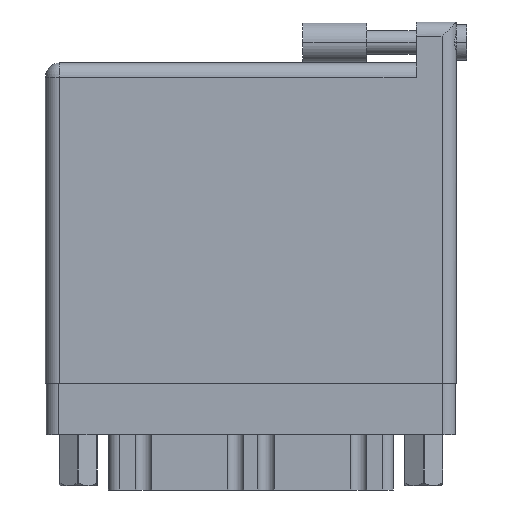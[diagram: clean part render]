
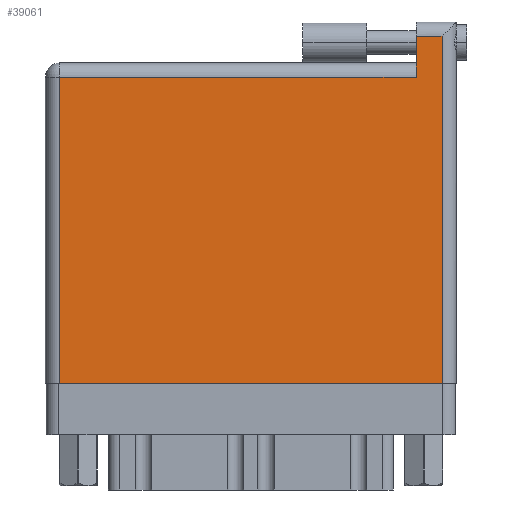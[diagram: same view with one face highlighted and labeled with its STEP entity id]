
A CAD part, front view. The second image highlights one B-rep face of the part: STEP entity #39061.
In plain terms, the highlighted face is planar.
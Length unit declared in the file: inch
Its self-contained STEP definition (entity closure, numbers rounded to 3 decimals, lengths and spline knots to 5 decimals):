
#5 = ORIENTED_EDGE ( 'NONE', *, *, #36815, .T. ) ;
#1291 = VERTEX_POINT ( 'NONE', #3061 ) ;
#2161 = VECTOR ( 'NONE', #46691, 39.37008 ) ;
#2641 = DIRECTION ( 'NONE',  ( -1., 0., 0. ) ) ;
#2986 = VECTOR ( 'NONE', #26670, 39.37008 ) ;
#3061 = CARTESIAN_POINT ( 'NONE',  ( 1.811, 1.496, 0. ) ) ;
#4085 = EDGE_CURVE ( 'NONE', #36814, #37633, #35829, .T. ) ;
#4167 = VERTEX_POINT ( 'NONE', #31505 ) ;
#5212 = EDGE_CURVE ( 'NONE', #37633, #35950, #10649, .T. ) ;
#6495 = ORIENTED_EDGE ( 'NONE', *, *, #18965, .T. ) ;
#6812 = CARTESIAN_POINT ( 'NONE',  ( 0., 0., 0. ) ) ;
#10148 = LINE ( 'NONE', #13484, #28667 ) ;
#10649 = LINE ( 'NONE', #6812, #2161 ) ;
#13034 = ORIENTED_EDGE ( 'NONE', *, *, #5212, .T. ) ;
#13484 = CARTESIAN_POINT ( 'NONE',  ( 1.938, 1.766, 0. ) ) ;
#13700 = LINE ( 'NONE', #32299, #39753 ) ;
#17679 = FACE_OUTER_BOUND ( 'NONE', #38819, .T. ) ;
#18419 = LINE ( 'NONE', #33679, #44116 ) ;
#18526 = EDGE_CURVE ( 'NONE', #35950, #4167, #10148, .T. ) ;
#18965 = EDGE_CURVE ( 'NONE', #1291, #36814, #13700, .T. ) ;
#19088 = CARTESIAN_POINT ( 'NONE',  ( 0.07, 0., 0. ) ) ;
#19485 = LINE ( 'NONE', #23302, #2986 ) ;
#21342 = DIRECTION ( 'NONE',  ( 0., 1., 0. ) ) ;
#23302 = CARTESIAN_POINT ( 'NONE',  ( 0., 1.696, 0. ) ) ;
#26670 = DIRECTION ( 'NONE',  ( -1., 0., 0. ) ) ;
#27756 = DIRECTION ( 'NONE',  ( -1., 0., 0. ) ) ;
#28126 = VERTEX_POINT ( 'NONE', #35622 ) ;
#28667 = VECTOR ( 'NONE', #21342, 39.37008 ) ;
#31330 = AXIS2_PLACEMENT_3D ( 'NONE', #43005, #46364, #2641 ) ;
#31355 = ORIENTED_EDGE ( 'NONE', *, *, #35654, .T. ) ;
#31505 = CARTESIAN_POINT ( 'NONE',  ( 1.938, 1.696, 0. ) ) ;
#32004 = DIRECTION ( 'NONE',  ( 0., -1., 0. ) ) ;
#32299 = CARTESIAN_POINT ( 'NONE',  ( 0., 1.496, 0. ) ) ;
#32982 = DIRECTION ( 'NONE',  ( 0., -1., 0. ) ) ;
#33679 = CARTESIAN_POINT ( 'NONE',  ( 1.811, 1.766, 0. ) ) ;
#34057 = CARTESIAN_POINT ( 'NONE',  ( 0.07, 1.496, 0. ) ) ;
#35358 = PLANE ( 'NONE',  #31330 ) ;
#35622 = CARTESIAN_POINT ( 'NONE',  ( 1.811, 1.696, 0. ) ) ;
#35654 = EDGE_CURVE ( 'NONE', #28126, #1291, #18419, .T. ) ;
#35829 = LINE ( 'NONE', #42751, #39534 ) ;
#35950 = VERTEX_POINT ( 'NONE', #38134 ) ;
#36814 = VERTEX_POINT ( 'NONE', #34057 ) ;
#36815 = EDGE_CURVE ( 'NONE', #4167, #28126, #19485, .T. ) ;
#37336 = ORIENTED_EDGE ( 'NONE', *, *, #4085, .T. ) ;
#37633 = VERTEX_POINT ( 'NONE', #19088 ) ;
#38134 = CARTESIAN_POINT ( 'NONE',  ( 1.938, 0., 0. ) ) ;
#38819 = EDGE_LOOP ( 'NONE', ( #13034, #44916, #5, #31355, #6495, #37336 ) ) ;
#39061 = ADVANCED_FACE ( 'NONE', ( #17679 ), #35358, .F. ) ;
#39534 = VECTOR ( 'NONE', #32004, 39.37008 ) ;
#39753 = VECTOR ( 'NONE', #27756, 39.37008 ) ;
#42751 = CARTESIAN_POINT ( 'NONE',  ( 0.07, 0., 0. ) ) ;
#43005 = CARTESIAN_POINT ( 'NONE',  ( 0., 1.566, 0. ) ) ;
#44116 = VECTOR ( 'NONE', #32982, 39.37008 ) ;
#44916 = ORIENTED_EDGE ( 'NONE', *, *, #18526, .T. ) ;
#46364 = DIRECTION ( 'NONE',  ( 0., 0., -1. ) ) ;
#46691 = DIRECTION ( 'NONE',  ( 1., 0., 0. ) ) ;
